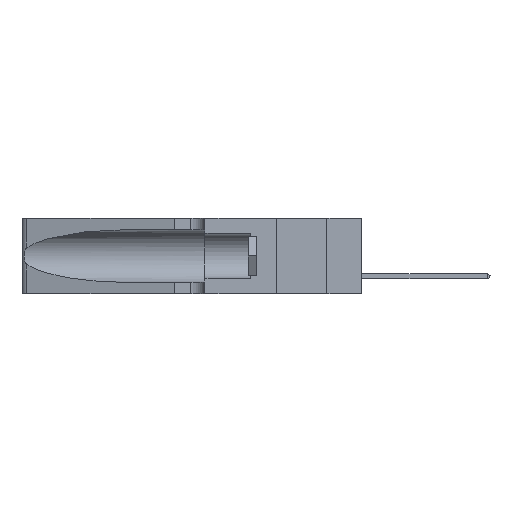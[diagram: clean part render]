
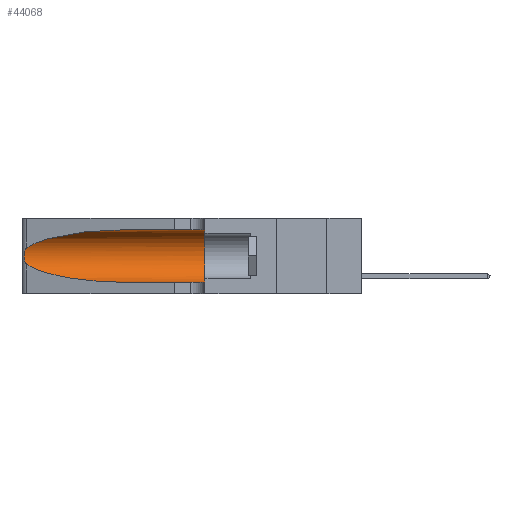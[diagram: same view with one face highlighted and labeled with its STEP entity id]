
A CAD part, left-side view. The second image highlights one B-rep face of the part: STEP entity #44068.
In plain terms, the highlighted cylindrical face has radius 3.308 mm (diameter 6.617 mm), a partial arc.
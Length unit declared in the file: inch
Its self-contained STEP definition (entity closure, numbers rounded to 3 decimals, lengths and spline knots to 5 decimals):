
#1393 = CARTESIAN_POINT ( 'NONE',  ( 0.1305, 0.35, 0.31525 ) ) ;
#2409 = CARTESIAN_POINT ( 'NONE',  ( 0.25789, 1.23486, 0.15765 ) ) ;
#2664 = ORIENTED_EDGE ( 'NONE', *, *, #27517, .F. ) ;
#2727 = CARTESIAN_POINT ( 'NONE',  ( 0.25487, 1.22718, 0.14631 ) ) ;
#3698 = CARTESIAN_POINT ( 'NONE',  ( 0.25487, 1.22718, 0.14631 ) ) ;
#4551 = EDGE_LOOP ( 'NONE', ( #43009, #9076, #21061, #40011, #30669, #2664 ) ) ;
#6128 = CARTESIAN_POINT ( 'NONE',  ( 0.26018, 1.23835, 0.19895 ) ) ;
#6269 = CARTESIAN_POINT ( 'NONE',  ( 0.25639, 1.23186, 0.15144 ) ) ;
#6602 = CARTESIAN_POINT ( 'NONE',  ( 0.25856, 1.23593, 0.16098 ) ) ;
#7735 = AXIS2_PLACEMENT_3D ( 'NONE', #12643, #34754, #16475 ) ;
#9076 = ORIENTED_EDGE ( 'NONE', *, *, #38563, .T. ) ;
#9777 = FACE_OUTER_BOUND ( 'NONE', #4551, .T. ) ;
#10056 = VECTOR ( 'NONE', #46447, 39.37008 ) ;
#10844 = CARTESIAN_POINT ( 'NONE',  ( 0.1305, 0.72297, 0.31525 ) ) ;
#11521 = CARTESIAN_POINT ( 'NONE',  ( 0.18966, 0.96281, 0.05475 ) ) ;
#12046 = CARTESIAN_POINT ( 'NONE',  ( 0.2373, 1.15595, 0.28018 ) ) ;
#12643 = CARTESIAN_POINT ( 'NONE',  ( 0.1305, 0.35, 0.185 ) ) ;
#13207 = CARTESIAN_POINT ( 'NONE',  ( 0.25487, 1.22718, 0.22369 ) ) ;
#13506 = CARTESIAN_POINT ( 'NONE',  ( 0.25487, 1.22718, 0.22369 ) ) ;
#14621 = LINE ( 'NONE', #42882, #16353 ) ;
#15809 = DIRECTION ( 'NONE',  ( 0., -1., 0. ) ) ;
#16203 = CARTESIAN_POINT ( 'NONE',  ( 0.1305, 0.72297, 0.31525 ) ) ;
#16353 = VECTOR ( 'NONE', #21850, 39.37008 ) ;
#16398 = AXIS2_PLACEMENT_3D ( 'NONE', #26733, #15809, #30740 ) ;
#16475 = DIRECTION ( 'NONE',  ( 0., 0., 1. ) ) ;
#17008 = CARTESIAN_POINT ( 'NONE',  ( 0.25555, 1.22994, 0.2215 ) ) ;
#17440 = EDGE_CURVE ( 'NONE', #17687, #36668, #42816, .T. ) ;
#17598 = CARTESIAN_POINT ( 'NONE',  ( 0.1305, 1.61858, 0.05475 ) ) ;
#17687 = VERTEX_POINT ( 'NONE', #1393 ) ;
#19555 = CARTESIAN_POINT ( 'NONE',  ( 0.18966, 0.96281, 0.31525 ) ) ;
#20300 = EDGE_CURVE ( 'NONE', #36033, #44977, #41931, .T. ) ;
#21061 = ORIENTED_EDGE ( 'NONE', *, *, #27939, .T. ) ;
#21850 = DIRECTION ( 'NONE',  ( 0., -1., 0. ) ) ;
#22216 = EDGE_CURVE ( 'NONE', #28268, #36668, #28979, .T. ) ;
#23972 = VERTEX_POINT ( 'NONE', #29127 ) ;
#24738 = CARTESIAN_POINT ( 'NONE',  ( 0.1305, 0.35, 0.05475 ) ) ;
#24864 = CARTESIAN_POINT ( 'NONE',  ( 0.26075, 1.23896, 0.178 ) ) ;
#26733 = CARTESIAN_POINT ( 'NONE',  ( 0.1305, 1.61858, 0.185 ) ) ;
#27517 = EDGE_CURVE ( 'NONE', #36033, #17687, #14621, .T. ) ;
#27936 = CARTESIAN_POINT ( 'NONE',  ( 0.25639, 1.23184, 0.21858 ) ) ;
#27939 = EDGE_CURVE ( 'NONE', #23972, #28268, #42787, .T. ) ;
#28268 = VERTEX_POINT ( 'NONE', #45485 ) ;
#28417 = CARTESIAN_POINT ( 'NONE',  ( 0.25555, 1.22993, 0.14849 ) ) ;
#28979 = LINE ( 'NONE', #17598, #10056 ) ;
#29127 = CARTESIAN_POINT ( 'NONE',  ( 0.25487, 1.22718, 0.14631 ) ) ;
#29825 = CARTESIAN_POINT ( 'NONE',  ( 0.1305, 0.72297, 0.05475 ) ) ;
#30669 = ORIENTED_EDGE ( 'NONE', *, *, #17440, .F. ) ;
#30740 = DIRECTION ( 'NONE',  ( 0., 0., -1. ) ) ;
#31333 = B_SPLINE_CURVE_WITH_KNOTS ( 'NONE', 3,
 ( #13506, #17008, #27936, #46166, #32069, #6128, #35599, #24864, #35288, #6602, #2409, #6269, #28417, #2727 ),
 .UNSPECIFIED., .F., .F.,
 ( 4, 2, 2, 2, 2, 2, 4 ),
 ( 0., 0.00027, 0.00053, 0.00107, 0.0016, 0.00187, 0.00214 ),
 .UNSPECIFIED. ) ;
#32069 = CARTESIAN_POINT ( 'NONE',  ( 0.25854, 1.2359, 0.20912 ) ) ;
#34754 = DIRECTION ( 'NONE',  ( 0., 1., 0. ) ) ;
#35288 = CARTESIAN_POINT ( 'NONE',  ( 0.26017, 1.23833, 0.17102 ) ) ;
#35599 = CARTESIAN_POINT ( 'NONE',  ( 0.26075, 1.23896, 0.19203 ) ) ;
#36033 = VERTEX_POINT ( 'NONE', #10844 ) ;
#36668 = VERTEX_POINT ( 'NONE', #24738 ) ;
#38563 = EDGE_CURVE ( 'NONE', #44977, #23972, #31333, .T. ) ;
#39012 = CYLINDRICAL_SURFACE ( 'NONE', #16398, 0.13025 ) ;
#40011 = ORIENTED_EDGE ( 'NONE', *, *, #22216, .T. ) ;
#41066 = CARTESIAN_POINT ( 'NONE',  ( 0.2373, 1.15595, 0.08982 ) ) ;
#41931 =( BOUNDED_CURVE ( )  B_SPLINE_CURVE ( 3, ( #16203, #19555, #12046, #45217 ),
 .UNSPECIFIED., .F., .F. ) 
 B_SPLINE_CURVE_WITH_KNOTS ( ( 4, 4 ),
 ( 1.5708, 2.84003 ),
 .UNSPECIFIED. ) 
 CURVE ( )  GEOMETRIC_REPRESENTATION_ITEM ( )  RATIONAL_B_SPLINE_CURVE ( ( 1., 0.87, 0.87, 1. ) ) 
 REPRESENTATION_ITEM ( '' )  );
#42787 =( BOUNDED_CURVE ( )  B_SPLINE_CURVE ( 3, ( #3698, #41066, #11521, #29825 ),
 .UNSPECIFIED., .F., .F. ) 
 B_SPLINE_CURVE_WITH_KNOTS ( ( 4, 4 ),
 ( 3.44316, 4.71239 ),
 .UNSPECIFIED. ) 
 CURVE ( )  GEOMETRIC_REPRESENTATION_ITEM ( )  RATIONAL_B_SPLINE_CURVE ( ( 1., 0.87, 0.87, 1. ) ) 
 REPRESENTATION_ITEM ( '' )  );
#42816 = CIRCLE ( 'NONE', #7735, 0.13025 ) ;
#42882 = CARTESIAN_POINT ( 'NONE',  ( 0.1305, 1.61858, 0.31525 ) ) ;
#43009 = ORIENTED_EDGE ( 'NONE', *, *, #20300, .T. ) ;
#44068 = ADVANCED_FACE ( 'NONE', ( #9777 ), #39012, .F. ) ;
#44977 = VERTEX_POINT ( 'NONE', #13207 ) ;
#45217 = CARTESIAN_POINT ( 'NONE',  ( 0.25487, 1.22718, 0.22369 ) ) ;
#45485 = CARTESIAN_POINT ( 'NONE',  ( 0.1305, 0.72297, 0.05475 ) ) ;
#46166 = CARTESIAN_POINT ( 'NONE',  ( 0.25787, 1.23484, 0.2124 ) ) ;
#46447 = DIRECTION ( 'NONE',  ( 0., -1., 0. ) ) ;
